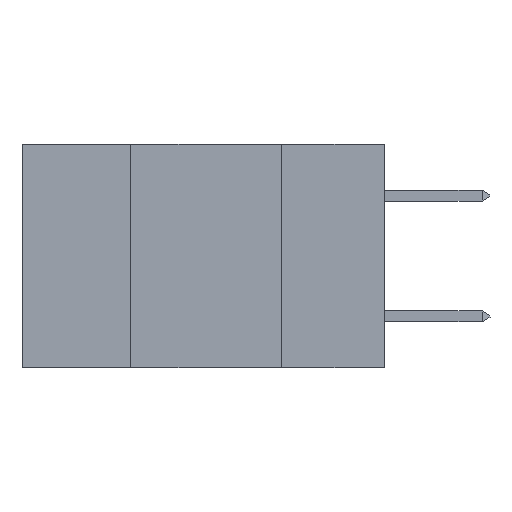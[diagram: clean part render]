
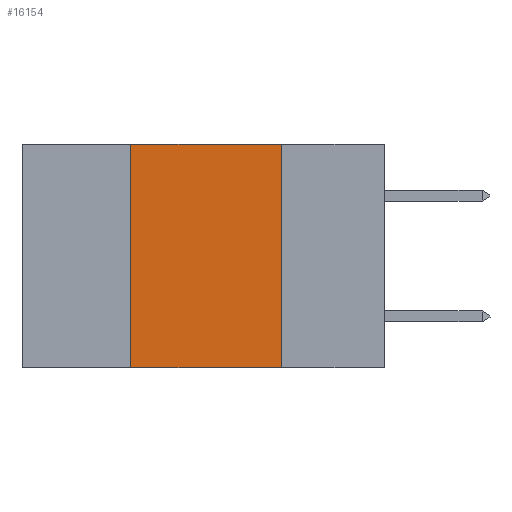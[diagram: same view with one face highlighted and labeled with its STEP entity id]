
A CAD part, left-side view. The second image highlights one B-rep face of the part: STEP entity #16154.
In plain terms, the highlighted planar face has unit normal (-1, 0, 0).
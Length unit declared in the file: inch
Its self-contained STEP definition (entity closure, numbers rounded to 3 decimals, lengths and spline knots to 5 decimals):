
#1152 = CARTESIAN_POINT ( 'NONE',  ( 0., 0.6, -0.37 ) ) ;
#2027 = CARTESIAN_POINT ( 'NONE',  ( 0., 0.42, -0.37 ) ) ;
#3145 = LINE ( 'NONE', #15286, #14660 ) ;
#3312 = DIRECTION ( 'NONE',  ( 0., -1., 0. ) ) ;
#3408 = CARTESIAN_POINT ( 'NONE',  ( 0., 0.17, 0. ) ) ;
#3442 = EDGE_CURVE ( 'NONE', #13788, #18758, #17013, .T. ) ;
#3605 = LINE ( 'NONE', #1152, #7171 ) ;
#4659 = ORIENTED_EDGE ( 'NONE', *, *, #6979, .F. ) ;
#4701 = ORIENTED_EDGE ( 'NONE', *, *, #17469, .F. ) ;
#4802 = ORIENTED_EDGE ( 'NONE', *, *, #3442, .F. ) ;
#4849 = ORIENTED_EDGE ( 'NONE', *, *, #19713, .T. ) ;
#5213 = DIRECTION ( 'NONE',  ( 0., 0., -1. ) ) ;
#5855 = PLANE ( 'NONE',  #6912 ) ;
#6912 = AXIS2_PLACEMENT_3D ( 'NONE', #19159, #9229, #20904 ) ;
#6979 = EDGE_CURVE ( 'NONE', #11411, #14931, #11279, .T. ) ;
#7171 = VECTOR ( 'NONE', #13249, 39.37008 ) ;
#7288 = FACE_OUTER_BOUND ( 'NONE', #17028, .T. ) ;
#7903 = CARTESIAN_POINT ( 'NONE',  ( 0., 0.17, 0. ) ) ;
#9229 = DIRECTION ( 'NONE',  ( 1., 0., 0. ) ) ;
#11279 = LINE ( 'NONE', #3408, #19126 ) ;
#11320 = CARTESIAN_POINT ( 'NONE',  ( 0., 0.42, 0. ) ) ;
#11411 = VERTEX_POINT ( 'NONE', #7903 ) ;
#12269 = CARTESIAN_POINT ( 'NONE',  ( 0., 0.17, -0.37 ) ) ;
#12520 = VECTOR ( 'NONE', #14782, 39.37008 ) ;
#13249 = DIRECTION ( 'NONE',  ( 0., -1., 0. ) ) ;
#13788 = VERTEX_POINT ( 'NONE', #2027 ) ;
#14056 = CARTESIAN_POINT ( 'NONE',  ( 0., 0.42, 0. ) ) ;
#14660 = VECTOR ( 'NONE', #3312, 39.37008 ) ;
#14782 = DIRECTION ( 'NONE',  ( 0., 0., 1. ) ) ;
#14931 = VERTEX_POINT ( 'NONE', #12269 ) ;
#15286 = CARTESIAN_POINT ( 'NONE',  ( 0., 0.6, 0. ) ) ;
#16154 = ADVANCED_FACE ( 'NONE', ( #7288 ), #5855, .F. ) ;
#17013 = LINE ( 'NONE', #11320, #12520 ) ;
#17028 = EDGE_LOOP ( 'NONE', ( #4659, #4701, #4802, #4849 ) ) ;
#17469 = EDGE_CURVE ( 'NONE', #18758, #11411, #3145, .T. ) ;
#18758 = VERTEX_POINT ( 'NONE', #14056 ) ;
#19126 = VECTOR ( 'NONE', #5213, 39.37008 ) ;
#19159 = CARTESIAN_POINT ( 'NONE',  ( 0., 0.6, 0. ) ) ;
#19713 = EDGE_CURVE ( 'NONE', #13788, #14931, #3605, .T. ) ;
#20904 = DIRECTION ( 'NONE',  ( 0., 0., -1. ) ) ;
